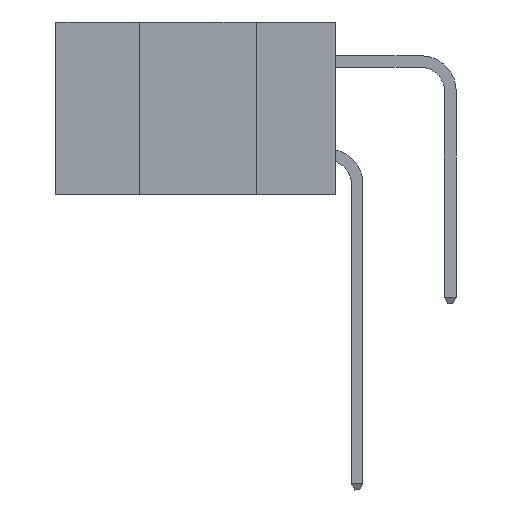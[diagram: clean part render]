
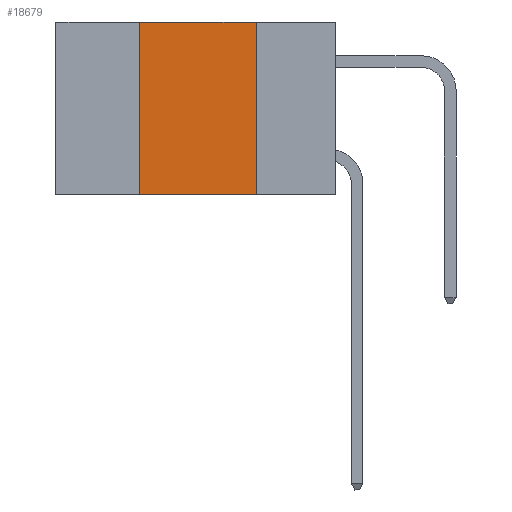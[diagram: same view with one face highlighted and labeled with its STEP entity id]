
A CAD part, left-side view. The second image highlights one B-rep face of the part: STEP entity #18679.
In plain terms, the highlighted planar face has unit normal (-1, 0, 0).
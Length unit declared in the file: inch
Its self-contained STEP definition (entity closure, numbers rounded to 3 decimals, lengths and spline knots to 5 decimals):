
#941 = ORIENTED_EDGE ( 'NONE', *, *, #21323, .T. ) ;
#1617 = CARTESIAN_POINT ( 'NONE',  ( 0., 0.6, 0. ) ) ;
#3059 = EDGE_CURVE ( 'NONE', #10219, #18147, #19683, .T. ) ;
#4042 = DIRECTION ( 'NONE',  ( 1., 0., 0. ) ) ;
#5107 = DIRECTION ( 'NONE',  ( 0., 0., 1. ) ) ;
#5842 = CARTESIAN_POINT ( 'NONE',  ( 0., 0.42, 0. ) ) ;
#6281 = CARTESIAN_POINT ( 'NONE',  ( 0., 0.42, 0. ) ) ;
#8734 = LINE ( 'NONE', #1617, #9692 ) ;
#8998 = VERTEX_POINT ( 'NONE', #14309 ) ;
#9692 = VECTOR ( 'NONE', #30123, 39.37008 ) ;
#10219 = VERTEX_POINT ( 'NONE', #27342 ) ;
#10266 = CARTESIAN_POINT ( 'NONE',  ( 0., 0.17, 0. ) ) ;
#11076 = ORIENTED_EDGE ( 'NONE', *, *, #15847, .F. ) ;
#12879 = VECTOR ( 'NONE', #5107, 39.37008 ) ;
#14309 = CARTESIAN_POINT ( 'NONE',  ( 0., 0.17, 0. ) ) ;
#15847 = EDGE_CURVE ( 'NONE', #18147, #8998, #8734, .T. ) ;
#16566 = FACE_OUTER_BOUND ( 'NONE', #21366, .T. ) ;
#16700 = EDGE_CURVE ( 'NONE', #8998, #25573, #20081, .T. ) ;
#18147 = VERTEX_POINT ( 'NONE', #6281 ) ;
#18679 = ADVANCED_FACE ( 'NONE', ( #16566 ), #21459, .F. ) ;
#18928 = DIRECTION ( 'NONE',  ( 0., 0., -1. ) ) ;
#19338 = ORIENTED_EDGE ( 'NONE', *, *, #3059, .F. ) ;
#19343 = AXIS2_PLACEMENT_3D ( 'NONE', #26062, #4042, #18928 ) ;
#19683 = LINE ( 'NONE', #5842, #12879 ) ;
#20081 = LINE ( 'NONE', #10266, #24391 ) ;
#21323 = EDGE_CURVE ( 'NONE', #10219, #25573, #24032, .T. ) ;
#21366 = EDGE_LOOP ( 'NONE', ( #25793, #11076, #19338, #941 ) ) ;
#21459 = PLANE ( 'NONE',  #19343 ) ;
#24032 = LINE ( 'NONE', #30679, #31092 ) ;
#24391 = VECTOR ( 'NONE', #29118, 39.37008 ) ;
#25573 = VERTEX_POINT ( 'NONE', #25839 ) ;
#25793 = ORIENTED_EDGE ( 'NONE', *, *, #16700, .F. ) ;
#25839 = CARTESIAN_POINT ( 'NONE',  ( 0., 0.17, -0.37 ) ) ;
#26062 = CARTESIAN_POINT ( 'NONE',  ( 0., 0.6, 0. ) ) ;
#27342 = CARTESIAN_POINT ( 'NONE',  ( 0., 0.42, -0.37 ) ) ;
#29118 = DIRECTION ( 'NONE',  ( 0., 0., -1. ) ) ;
#30123 = DIRECTION ( 'NONE',  ( 0., -1., 0. ) ) ;
#30679 = CARTESIAN_POINT ( 'NONE',  ( 0., 0.6, -0.37 ) ) ;
#30995 = DIRECTION ( 'NONE',  ( 0., -1., 0. ) ) ;
#31092 = VECTOR ( 'NONE', #30995, 39.37008 ) ;
